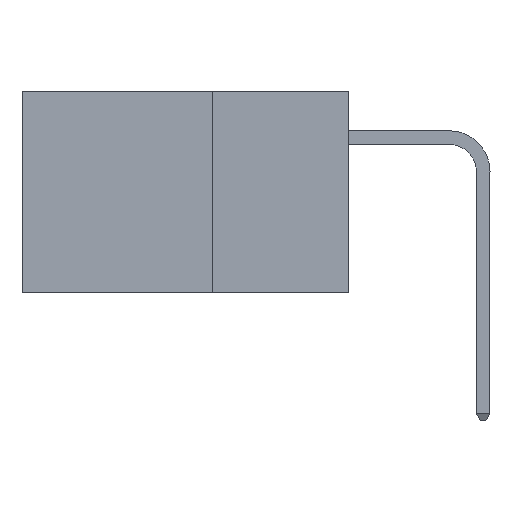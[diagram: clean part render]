
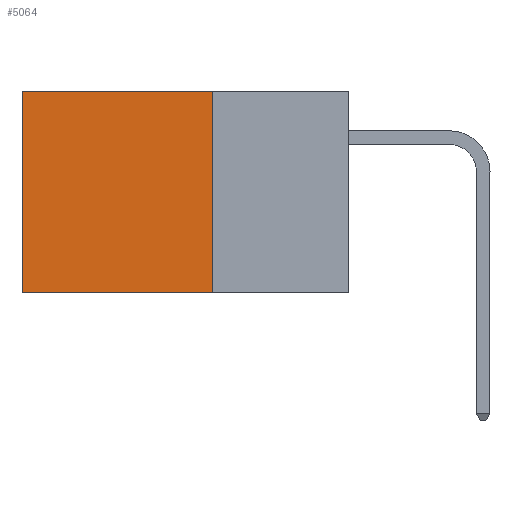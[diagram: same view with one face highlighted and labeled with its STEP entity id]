
A CAD part, left-side view. The second image highlights one B-rep face of the part: STEP entity #5064.
In plain terms, the highlighted planar face has unit normal (-1, 0, 0).
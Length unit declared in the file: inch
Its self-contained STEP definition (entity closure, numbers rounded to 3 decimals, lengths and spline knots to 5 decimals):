
#42 = PLANE ( 'NONE',  #7924 ) ;
#259 = VECTOR ( 'NONE', #10012, 39.37008 ) ;
#345 = EDGE_CURVE ( 'NONE', #3334, #6392, #8743, .T. ) ;
#724 = VERTEX_POINT ( 'NONE', #6744 ) ;
#1669 = LINE ( 'NONE', #6034, #4701 ) ;
#2255 = ORIENTED_EDGE ( 'NONE', *, *, #345, .T. ) ;
#2377 = DIRECTION ( 'NONE',  ( 0., 0., -1. ) ) ;
#2597 = CARTESIAN_POINT ( 'NONE',  ( 0.2875, 0.25, 0. ) ) ;
#3198 = EDGE_CURVE ( 'NONE', #4687, #724, #1669, .T. ) ;
#3236 = CARTESIAN_POINT ( 'NONE',  ( 0.2875, 0.6, 0. ) ) ;
#3293 = EDGE_CURVE ( 'NONE', #4687, #3334, #6746, .T. ) ;
#3334 = VERTEX_POINT ( 'NONE', #3236 ) ;
#3348 = EDGE_LOOP ( 'NONE', ( #2255, #3532, #5226, #9724 ) ) ;
#3532 = ORIENTED_EDGE ( 'NONE', *, *, #8476, .F. ) ;
#3881 = CARTESIAN_POINT ( 'NONE',  ( 0.2875, 0.25, 0. ) ) ;
#4594 = CARTESIAN_POINT ( 'NONE',  ( 0.2875, 0.6, 0. ) ) ;
#4687 = VERTEX_POINT ( 'NONE', #2597 ) ;
#4701 = VECTOR ( 'NONE', #6802, 39.37008 ) ;
#5064 = ADVANCED_FACE ( 'NONE', ( #9557 ), #42, .F. ) ;
#5226 = ORIENTED_EDGE ( 'NONE', *, *, #3198, .F. ) ;
#5454 = CARTESIAN_POINT ( 'NONE',  ( 0.2875, 0.25, 0. ) ) ;
#5772 = CARTESIAN_POINT ( 'NONE',  ( 0.2875, 0.25, -0.37 ) ) ;
#6034 = CARTESIAN_POINT ( 'NONE',  ( 0.2875, 0.25, 0. ) ) ;
#6392 = VERTEX_POINT ( 'NONE', #9871 ) ;
#6744 = CARTESIAN_POINT ( 'NONE',  ( 0.2875, 0.25, -0.37 ) ) ;
#6746 = LINE ( 'NONE', #3881, #7978 ) ;
#6802 = DIRECTION ( 'NONE',  ( 0., 0., -1. ) ) ;
#6982 = DIRECTION ( 'NONE',  ( 1., 0., 0. ) ) ;
#7299 = VECTOR ( 'NONE', #9655, 39.37008 ) ;
#7792 = DIRECTION ( 'NONE',  ( 0., 1., 0. ) ) ;
#7924 = AXIS2_PLACEMENT_3D ( 'NONE', #5454, #6982, #2377 ) ;
#7978 = VECTOR ( 'NONE', #7792, 39.37008 ) ;
#8165 = LINE ( 'NONE', #5772, #7299 ) ;
#8476 = EDGE_CURVE ( 'NONE', #724, #6392, #8165, .T. ) ;
#8743 = LINE ( 'NONE', #4594, #259 ) ;
#9557 = FACE_OUTER_BOUND ( 'NONE', #3348, .T. ) ;
#9655 = DIRECTION ( 'NONE',  ( 0., 1., 0. ) ) ;
#9724 = ORIENTED_EDGE ( 'NONE', *, *, #3293, .T. ) ;
#9871 = CARTESIAN_POINT ( 'NONE',  ( 0.2875, 0.6, -0.37 ) ) ;
#10012 = DIRECTION ( 'NONE',  ( 0., 0., -1. ) ) ;
